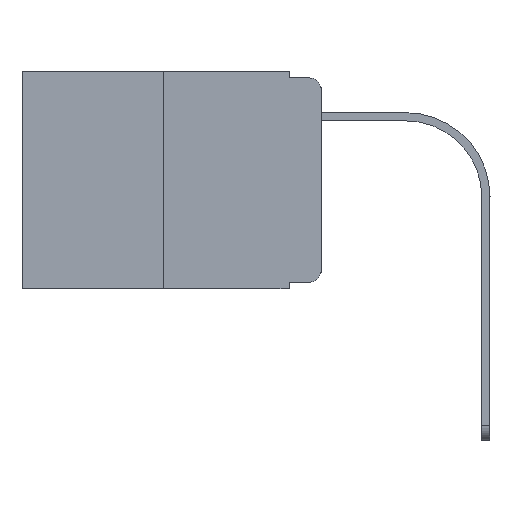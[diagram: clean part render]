
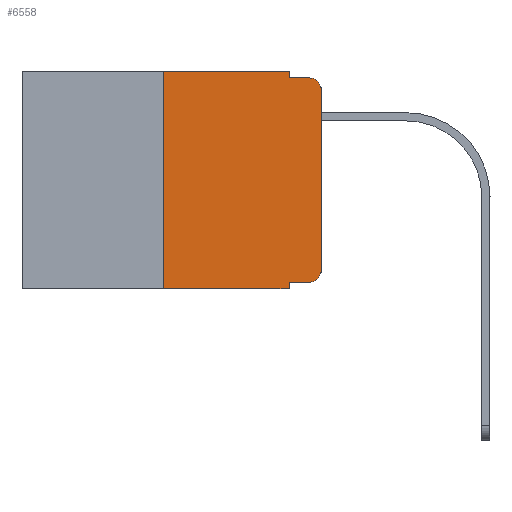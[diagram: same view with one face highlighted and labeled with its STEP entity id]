
A CAD part, left-side view. The second image highlights one B-rep face of the part: STEP entity #6558.
In plain terms, the highlighted planar face has unit normal (-1, 0, 0).
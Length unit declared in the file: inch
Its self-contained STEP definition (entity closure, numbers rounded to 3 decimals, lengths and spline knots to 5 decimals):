
#173 = VECTOR ( 'NONE', #799, 39.37008 ) ;
#264 = CARTESIAN_POINT ( 'NONE',  ( 0., 0.051, -0.01 ) ) ;
#370 = DIRECTION ( 'NONE',  ( 0., 0., -1. ) ) ;
#572 = ORIENTED_EDGE ( 'NONE', *, *, #4322, .T. ) ;
#694 = CARTESIAN_POINT ( 'NONE',  ( 0., 0., -0.03 ) ) ;
#799 = DIRECTION ( 'NONE',  ( 0., 0., -1. ) ) ;
#1101 = DIRECTION ( 'NONE',  ( 1., 0., 0. ) ) ;
#1233 = DIRECTION ( 'NONE',  ( -1., 0., 0. ) ) ;
#1398 = VECTOR ( 'NONE', #7655, 39.37008 ) ;
#1641 = VECTOR ( 'NONE', #9344, 39.37008 ) ;
#1755 = VERTEX_POINT ( 'NONE', #2762 ) ;
#1797 = CARTESIAN_POINT ( 'NONE',  ( 0., 0.051, -0.343 ) ) ;
#2054 = EDGE_CURVE ( 'NONE', #10005, #7563, #5887, .T. ) ;
#2095 = EDGE_CURVE ( 'NONE', #9093, #5083, #5903, .T. ) ;
#2126 = LINE ( 'NONE', #264, #2353 ) ;
#2245 = DIRECTION ( 'NONE',  ( 0., 0., 1. ) ) ;
#2349 = ORIENTED_EDGE ( 'NONE', *, *, #8960, .F. ) ;
#2353 = VECTOR ( 'NONE', #3810, 39.37008 ) ;
#2762 = CARTESIAN_POINT ( 'NONE',  ( 0., 0.02, -0.333 ) ) ;
#3041 = CARTESIAN_POINT ( 'NONE',  ( 0., 0., 0. ) ) ;
#3056 = CARTESIAN_POINT ( 'NONE',  ( 0., 0.25, 0. ) ) ;
#3261 = CARTESIAN_POINT ( 'NONE',  ( 0., 0.02, -0.03 ) ) ;
#3283 = CARTESIAN_POINT ( 'NONE',  ( 0., 0.051, 0. ) ) ;
#3309 = CARTESIAN_POINT ( 'NONE',  ( 0., 0.051, -0.01 ) ) ;
#3454 = VECTOR ( 'NONE', #2245, 39.37008 ) ;
#3493 = CARTESIAN_POINT ( 'NONE',  ( 0., 0.051, -0.333 ) ) ;
#3543 = ORIENTED_EDGE ( 'NONE', *, *, #8157, .F. ) ;
#3637 = CARTESIAN_POINT ( 'NONE',  ( 0., 0.25, 0. ) ) ;
#3667 = VERTEX_POINT ( 'NONE', #7486 ) ;
#3810 = DIRECTION ( 'NONE',  ( 0., -1., 0. ) ) ;
#3813 = LINE ( 'NONE', #3041, #3454 ) ;
#4322 = EDGE_CURVE ( 'NONE', #7609, #1755, #5022, .T. ) ;
#4536 = LINE ( 'NONE', #6308, #7751 ) ;
#4589 = ORIENTED_EDGE ( 'NONE', *, *, #7174, .F. ) ;
#5022 = LINE ( 'NONE', #7968, #1641 ) ;
#5083 = VERTEX_POINT ( 'NONE', #5898 ) ;
#5382 = CARTESIAN_POINT ( 'NONE',  ( 0., 0.473, 0. ) ) ;
#5509 = DIRECTION ( 'NONE',  ( 0., -1., 0. ) ) ;
#5764 = CIRCLE ( 'NONE', #7391, 0.02 ) ;
#5887 = CIRCLE ( 'NONE', #8770, 0.02 ) ;
#5898 = CARTESIAN_POINT ( 'NONE',  ( 0., 0.051, 0. ) ) ;
#5903 = LINE ( 'NONE', #10223, #1398 ) ;
#5935 = DIRECTION ( 'NONE',  ( 0., 0., -1. ) ) ;
#6290 = VERTEX_POINT ( 'NONE', #3309 ) ;
#6308 = CARTESIAN_POINT ( 'NONE',  ( 0., 0.473, -0.343 ) ) ;
#6558 = ADVANCED_FACE ( 'NONE', ( #10590 ), #10762, .F. ) ;
#6606 = EDGE_CURVE ( 'NONE', #9658, #9093, #8056, .T. ) ;
#6694 = DIRECTION ( 'NONE',  ( 0., 0., -1. ) ) ;
#7057 = EDGE_LOOP ( 'NONE', ( #7426, #10355, #3543, #4589, #7456, #10119, #8825, #2349, #572, #8840 ) ) ;
#7174 = EDGE_CURVE ( 'NONE', #5083, #6290, #9510, .T. ) ;
#7391 = AXIS2_PLACEMENT_3D ( 'NONE', #10663, #1233, #9841 ) ;
#7426 = ORIENTED_EDGE ( 'NONE', *, *, #9469, .T. ) ;
#7456 = ORIENTED_EDGE ( 'NONE', *, *, #2095, .F. ) ;
#7486 = CARTESIAN_POINT ( 'NONE',  ( 0., 0., -0.313 ) ) ;
#7563 = VERTEX_POINT ( 'NONE', #9668 ) ;
#7571 = VERTEX_POINT ( 'NONE', #1797 ) ;
#7609 = VERTEX_POINT ( 'NONE', #3493 ) ;
#7655 = DIRECTION ( 'NONE',  ( 0., -1., 0. ) ) ;
#7710 = DIRECTION ( 'NONE',  ( -1., 0., 0. ) ) ;
#7722 = EDGE_CURVE ( 'NONE', #1755, #3667, #5764, .T. ) ;
#7751 = VECTOR ( 'NONE', #5509, 39.37008 ) ;
#7968 = CARTESIAN_POINT ( 'NONE',  ( 0., 0.051, -0.333 ) ) ;
#8056 = LINE ( 'NONE', #3637, #8166 ) ;
#8157 = EDGE_CURVE ( 'NONE', #6290, #7563, #2126, .T. ) ;
#8166 = VECTOR ( 'NONE', #9826, 39.37008 ) ;
#8174 = EDGE_CURVE ( 'NONE', #9658, #7571, #4536, .T. ) ;
#8680 = VECTOR ( 'NONE', #5935, 39.37008 ) ;
#8770 = AXIS2_PLACEMENT_3D ( 'NONE', #3261, #7710, #6694 ) ;
#8825 = ORIENTED_EDGE ( 'NONE', *, *, #8174, .T. ) ;
#8840 = ORIENTED_EDGE ( 'NONE', *, *, #7722, .T. ) ;
#8960 = EDGE_CURVE ( 'NONE', #7609, #7571, #9516, .T. ) ;
#9093 = VERTEX_POINT ( 'NONE', #3056 ) ;
#9344 = DIRECTION ( 'NONE',  ( 0., -1., 0. ) ) ;
#9469 = EDGE_CURVE ( 'NONE', #3667, #10005, #3813, .T. ) ;
#9510 = LINE ( 'NONE', #3283, #173 ) ;
#9516 = LINE ( 'NONE', #11083, #8680 ) ;
#9658 = VERTEX_POINT ( 'NONE', #11041 ) ;
#9668 = CARTESIAN_POINT ( 'NONE',  ( 0., 0.02, -0.01 ) ) ;
#9804 = AXIS2_PLACEMENT_3D ( 'NONE', #5382, #1101, #370 ) ;
#9826 = DIRECTION ( 'NONE',  ( 0., 0., 1. ) ) ;
#9841 = DIRECTION ( 'NONE',  ( 0., 0., -1. ) ) ;
#10005 = VERTEX_POINT ( 'NONE', #694 ) ;
#10119 = ORIENTED_EDGE ( 'NONE', *, *, #6606, .F. ) ;
#10223 = CARTESIAN_POINT ( 'NONE',  ( 0., 0.473, 0. ) ) ;
#10355 = ORIENTED_EDGE ( 'NONE', *, *, #2054, .T. ) ;
#10590 = FACE_OUTER_BOUND ( 'NONE', #7057, .T. ) ;
#10663 = CARTESIAN_POINT ( 'NONE',  ( 0., 0.02, -0.313 ) ) ;
#10762 = PLANE ( 'NONE',  #9804 ) ;
#11041 = CARTESIAN_POINT ( 'NONE',  ( 0., 0.25, -0.343 ) ) ;
#11083 = CARTESIAN_POINT ( 'NONE',  ( 0., 0.051, 0. ) ) ;
